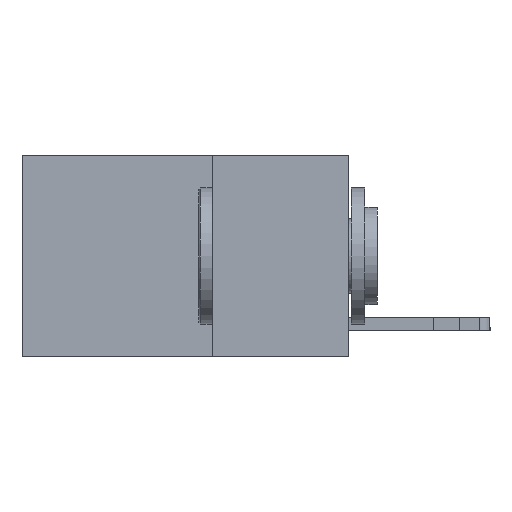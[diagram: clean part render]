
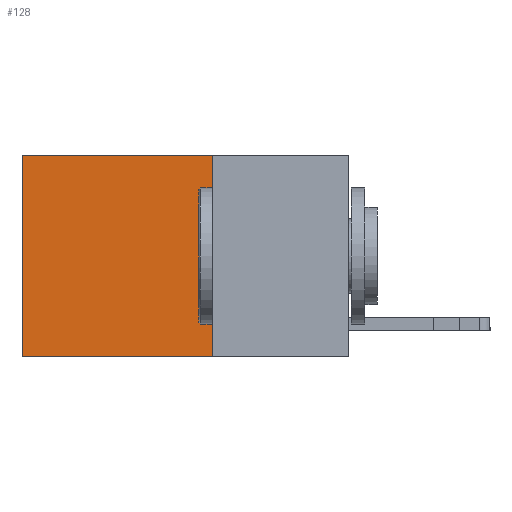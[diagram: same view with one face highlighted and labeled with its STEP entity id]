
A CAD part, left-side view. The second image highlights one B-rep face of the part: STEP entity #128.
In plain terms, the highlighted planar face has unit normal (-1, 0, 0).
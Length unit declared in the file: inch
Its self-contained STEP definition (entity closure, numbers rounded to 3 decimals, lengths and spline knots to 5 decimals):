
#128 = ADVANCED_FACE ( 'NONE', ( #5148 ), #13058, .F. ) ;
#570 = DIRECTION ( 'NONE',  ( 0., 0., -1. ) ) ;
#1007 = CARTESIAN_POINT ( 'NONE',  ( 0.2625, 0.6, 0. ) ) ;
#1125 = LINE ( 'NONE', #13057, #21972 ) ;
#1361 = VERTEX_POINT ( 'NONE', #1007 ) ;
#1679 = VERTEX_POINT ( 'NONE', #8135 ) ;
#1704 = LINE ( 'NONE', #7689, #23272 ) ;
#1794 = VECTOR ( 'NONE', #14866, 39.37008 ) ;
#2029 = VERTEX_POINT ( 'NONE', #5888 ) ;
#3191 = CARTESIAN_POINT ( 'NONE',  ( 0.2625, 0.25, 0. ) ) ;
#3799 = DIRECTION ( 'NONE',  ( 0., 0., -1. ) ) ;
#5148 = FACE_OUTER_BOUND ( 'NONE', #17884, .T. ) ;
#5888 = CARTESIAN_POINT ( 'NONE',  ( 0.2625, 0.6, -0.37 ) ) ;
#7283 = CARTESIAN_POINT ( 'NONE',  ( 0.2625, 0.25, 0. ) ) ;
#7686 = VERTEX_POINT ( 'NONE', #7283 ) ;
#7689 = CARTESIAN_POINT ( 'NONE',  ( 0.2625, 0.6, 0. ) ) ;
#8099 = ORIENTED_EDGE ( 'NONE', *, *, #18997, .F. ) ;
#8135 = CARTESIAN_POINT ( 'NONE',  ( 0.2625, 0.25, -0.37 ) ) ;
#8799 = DIRECTION ( 'NONE',  ( 0., 0., -1. ) ) ;
#9143 = CARTESIAN_POINT ( 'NONE',  ( 0.2625, 0.25, 0. ) ) ;
#11325 = LINE ( 'NONE', #9143, #1794 ) ;
#13057 = CARTESIAN_POINT ( 'NONE',  ( 0.2625, 0.25, -0.37 ) ) ;
#13058 = PLANE ( 'NONE',  #13673 ) ;
#13193 = EDGE_CURVE ( 'NONE', #1361, #2029, #1704, .T. ) ;
#13673 = AXIS2_PLACEMENT_3D ( 'NONE', #3191, #23093, #8799 ) ;
#14328 = CARTESIAN_POINT ( 'NONE',  ( 0.2625, 0.25, 0. ) ) ;
#14449 = ORIENTED_EDGE ( 'NONE', *, *, #17722, .F. ) ;
#14866 = DIRECTION ( 'NONE',  ( 0., 1., 0. ) ) ;
#14896 = DIRECTION ( 'NONE',  ( 0., 1., 0. ) ) ;
#15531 = ORIENTED_EDGE ( 'NONE', *, *, #16153, .T. ) ;
#16153 = EDGE_CURVE ( 'NONE', #7686, #1361, #11325, .T. ) ;
#17722 = EDGE_CURVE ( 'NONE', #7686, #1679, #20579, .T. ) ;
#17884 = EDGE_LOOP ( 'NONE', ( #21400, #8099, #14449, #15531 ) ) ;
#18997 = EDGE_CURVE ( 'NONE', #1679, #2029, #1125, .T. ) ;
#20344 = VECTOR ( 'NONE', #570, 39.37008 ) ;
#20579 = LINE ( 'NONE', #14328, #20344 ) ;
#21400 = ORIENTED_EDGE ( 'NONE', *, *, #13193, .T. ) ;
#21972 = VECTOR ( 'NONE', #14896, 39.37008 ) ;
#23093 = DIRECTION ( 'NONE',  ( 1., 0., 0. ) ) ;
#23272 = VECTOR ( 'NONE', #3799, 39.37008 ) ;
